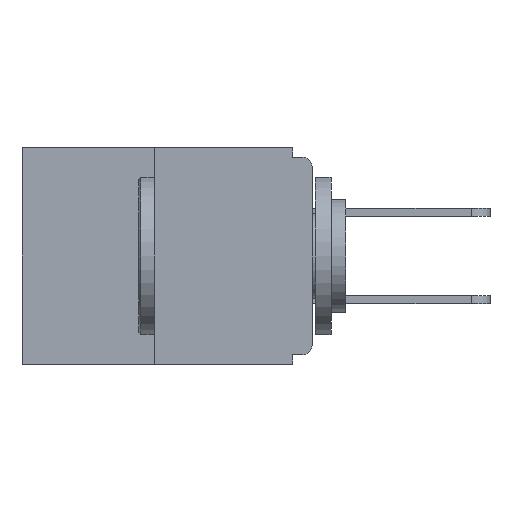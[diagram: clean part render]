
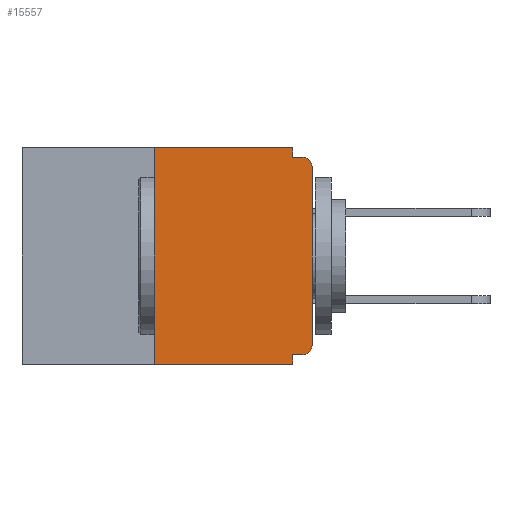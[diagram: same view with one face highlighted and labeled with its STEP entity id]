
A CAD part, left-side view. The second image highlights one B-rep face of the part: STEP entity #15557.
In plain terms, the highlighted planar face has unit normal (-1, 0, 0).
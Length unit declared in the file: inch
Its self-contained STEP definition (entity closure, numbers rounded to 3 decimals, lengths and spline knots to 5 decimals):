
#35 = VECTOR ( 'NONE', #12856, 39.37008 ) ;
#176 = CARTESIAN_POINT ( 'NONE',  ( 0., 0.46, -0.343 ) ) ;
#621 = EDGE_CURVE ( 'NONE', #2113, #1861, #16012, .T. ) ;
#1247 = AXIS2_PLACEMENT_3D ( 'NONE', #16450, #9377, #10762 ) ;
#1273 = CARTESIAN_POINT ( 'NONE',  ( 0., 0.031, 0. ) ) ;
#1492 = LINE ( 'NONE', #2954, #9664 ) ;
#1861 = VERTEX_POINT ( 'NONE', #2245 ) ;
#2043 = ORIENTED_EDGE ( 'NONE', *, *, #13048, .F. ) ;
#2113 = VERTEX_POINT ( 'NONE', #16400 ) ;
#2144 = DIRECTION ( 'NONE',  ( 0., 0., 1. ) ) ;
#2245 = CARTESIAN_POINT ( 'NONE',  ( 0., 0.25, 0. ) ) ;
#2322 = LINE ( 'NONE', #176, #35 ) ;
#2711 = DIRECTION ( 'NONE',  ( 0., 0., -1. ) ) ;
#2718 = VERTEX_POINT ( 'NONE', #10577 ) ;
#2741 = VECTOR ( 'NONE', #3074, 39.37008 ) ;
#2856 = EDGE_CURVE ( 'NONE', #17832, #16811, #10624, .T. ) ;
#2954 = CARTESIAN_POINT ( 'NONE',  ( 0., 0.031, -0.343 ) ) ;
#3074 = DIRECTION ( 'NONE',  ( 0., 1., 0. ) ) ;
#3161 = LINE ( 'NONE', #1273, #17368 ) ;
#3874 = EDGE_CURVE ( 'NONE', #2113, #8881, #2322, .T. ) ;
#4319 = EDGE_CURVE ( 'NONE', #7354, #10038, #17182, .T. ) ;
#4588 = ORIENTED_EDGE ( 'NONE', *, *, #4615, .F. ) ;
#4615 = EDGE_CURVE ( 'NONE', #17832, #2718, #12153, .T. ) ;
#4769 = EDGE_CURVE ( 'NONE', #2718, #8881, #1492, .T. ) ;
#4914 = LINE ( 'NONE', #5307, #12303 ) ;
#5307 = CARTESIAN_POINT ( 'NONE',  ( 0., 0., 0. ) ) ;
#5492 = VECTOR ( 'NONE', #18393, 39.37008 ) ;
#5916 = VERTEX_POINT ( 'NONE', #18441 ) ;
#6163 = DIRECTION ( 'NONE',  ( 0., 0., -1. ) ) ;
#6307 = DIRECTION ( 'NONE',  ( 0., -1., 0. ) ) ;
#7354 = VERTEX_POINT ( 'NONE', #9863 ) ;
#7392 = CARTESIAN_POINT ( 'NONE',  ( 0., 0., -0.328 ) ) ;
#7546 = ORIENTED_EDGE ( 'NONE', *, *, #2856, .T. ) ;
#7665 = ORIENTED_EDGE ( 'NONE', *, *, #16874, .T. ) ;
#8080 = CARTESIAN_POINT ( 'NONE',  ( 0., 0.015, -0.313 ) ) ;
#8425 = VECTOR ( 'NONE', #6307, 39.37008 ) ;
#8881 = VERTEX_POINT ( 'NONE', #14067 ) ;
#9003 = AXIS2_PLACEMENT_3D ( 'NONE', #14749, #16465, #6163 ) ;
#9315 = LINE ( 'NONE', #13408, #8425 ) ;
#9377 = DIRECTION ( 'NONE',  ( 1., 0., 0. ) ) ;
#9664 = VECTOR ( 'NONE', #2711, 39.37008 ) ;
#9863 = CARTESIAN_POINT ( 'NONE',  ( 0., 0.031, -0.015 ) ) ;
#9871 = AXIS2_PLACEMENT_3D ( 'NONE', #8080, #10769, #12209 ) ;
#9965 = EDGE_CURVE ( 'NONE', #1861, #10956, #9315, .T. ) ;
#10038 = VERTEX_POINT ( 'NONE', #13847 ) ;
#10577 = CARTESIAN_POINT ( 'NONE',  ( 0., 0.031, -0.328 ) ) ;
#10624 = CIRCLE ( 'NONE', #9871, 0.015 ) ;
#10762 = DIRECTION ( 'NONE',  ( 0., 0., -1. ) ) ;
#10769 = DIRECTION ( 'NONE',  ( -1., 0., 0. ) ) ;
#10956 = VERTEX_POINT ( 'NONE', #17666 ) ;
#10982 = CARTESIAN_POINT ( 'NONE',  ( 0., 0., -0.015 ) ) ;
#11092 = EDGE_CURVE ( 'NONE', #5916, #10038, #12653, .T. ) ;
#11765 = ORIENTED_EDGE ( 'NONE', *, *, #9965, .F. ) ;
#12153 = LINE ( 'NONE', #7392, #2741 ) ;
#12209 = DIRECTION ( 'NONE',  ( 0., 0., -1. ) ) ;
#12303 = VECTOR ( 'NONE', #2144, 39.37008 ) ;
#12315 = CARTESIAN_POINT ( 'NONE',  ( 0., 0.25, 0. ) ) ;
#12653 = CIRCLE ( 'NONE', #9003, 0.015 ) ;
#12856 = DIRECTION ( 'NONE',  ( 0., -1., 0. ) ) ;
#13048 = EDGE_CURVE ( 'NONE', #10956, #7354, #3161, .T. ) ;
#13408 = CARTESIAN_POINT ( 'NONE',  ( 0., 0.46, 0. ) ) ;
#13544 = ORIENTED_EDGE ( 'NONE', *, *, #3874, .T. ) ;
#13847 = CARTESIAN_POINT ( 'NONE',  ( 0., 0.015, -0.015 ) ) ;
#13932 = DIRECTION ( 'NONE',  ( 0., 0., 1. ) ) ;
#14067 = CARTESIAN_POINT ( 'NONE',  ( 0., 0.031, -0.343 ) ) ;
#14749 = CARTESIAN_POINT ( 'NONE',  ( 0., 0.015, -0.03 ) ) ;
#14964 = EDGE_LOOP ( 'NONE', ( #11765, #16441, #13544, #15161, #4588, #7546, #7665, #18646, #16784, #2043 ) ) ;
#15161 = ORIENTED_EDGE ( 'NONE', *, *, #4769, .F. ) ;
#15266 = CARTESIAN_POINT ( 'NONE',  ( 0., 0., -0.313 ) ) ;
#15557 = ADVANCED_FACE ( 'NONE', ( #17795 ), #16512, .F. ) ;
#16012 = LINE ( 'NONE', #12315, #16935 ) ;
#16400 = CARTESIAN_POINT ( 'NONE',  ( 0., 0.25, -0.343 ) ) ;
#16441 = ORIENTED_EDGE ( 'NONE', *, *, #621, .F. ) ;
#16450 = CARTESIAN_POINT ( 'NONE',  ( 0., 0.46, 0. ) ) ;
#16465 = DIRECTION ( 'NONE',  ( -1., 0., 0. ) ) ;
#16512 = PLANE ( 'NONE',  #1247 ) ;
#16784 = ORIENTED_EDGE ( 'NONE', *, *, #4319, .F. ) ;
#16811 = VERTEX_POINT ( 'NONE', #15266 ) ;
#16874 = EDGE_CURVE ( 'NONE', #16811, #5916, #4914, .T. ) ;
#16935 = VECTOR ( 'NONE', #13932, 39.37008 ) ;
#17143 = CARTESIAN_POINT ( 'NONE',  ( 0., 0.015, -0.328 ) ) ;
#17182 = LINE ( 'NONE', #10982, #5492 ) ;
#17368 = VECTOR ( 'NONE', #18486, 39.37008 ) ;
#17666 = CARTESIAN_POINT ( 'NONE',  ( 0., 0.031, 0. ) ) ;
#17795 = FACE_OUTER_BOUND ( 'NONE', #14964, .T. ) ;
#17832 = VERTEX_POINT ( 'NONE', #17143 ) ;
#18393 = DIRECTION ( 'NONE',  ( 0., -1., 0. ) ) ;
#18441 = CARTESIAN_POINT ( 'NONE',  ( 0., 0., -0.03 ) ) ;
#18486 = DIRECTION ( 'NONE',  ( 0., 0., -1. ) ) ;
#18646 = ORIENTED_EDGE ( 'NONE', *, *, #11092, .T. ) ;
